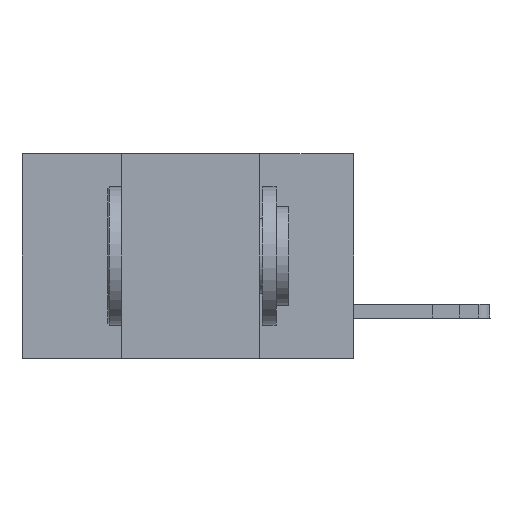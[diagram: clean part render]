
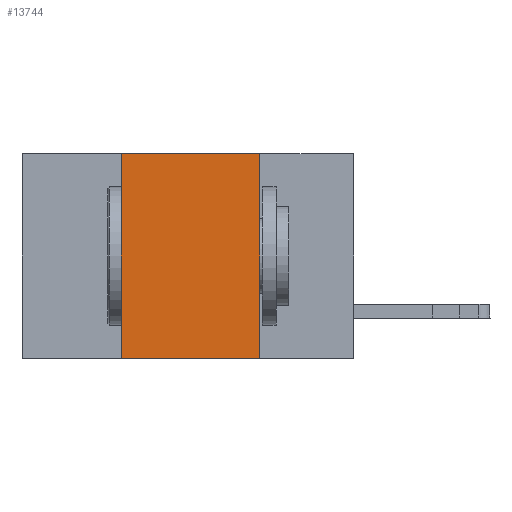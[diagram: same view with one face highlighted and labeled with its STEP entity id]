
A CAD part, left-side view. The second image highlights one B-rep face of the part: STEP entity #13744.
In plain terms, the highlighted planar face has unit normal (-1, 0, 0).
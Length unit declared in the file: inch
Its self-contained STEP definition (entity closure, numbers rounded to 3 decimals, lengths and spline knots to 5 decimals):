
#202 = VECTOR ( 'NONE', #1942, 39.37008 ) ;
#573 = VERTEX_POINT ( 'NONE', #10098 ) ;
#1404 = VECTOR ( 'NONE', #19814, 39.37008 ) ;
#1531 = DIRECTION ( 'NONE',  ( 0., 0., -1. ) ) ;
#1942 = DIRECTION ( 'NONE',  ( 0., 0., -1. ) ) ;
#2146 = LINE ( 'NONE', #12635, #4744 ) ;
#2466 = AXIS2_PLACEMENT_3D ( 'NONE', #9143, #10823, #1531 ) ;
#3136 = CARTESIAN_POINT ( 'NONE',  ( 0., 0.42, -0.37 ) ) ;
#3444 = EDGE_CURVE ( 'NONE', #18048, #16269, #6914, .T. ) ;
#4387 = LINE ( 'NONE', #14983, #10400 ) ;
#4631 = ORIENTED_EDGE ( 'NONE', *, *, #19738, .T. ) ;
#4744 = VECTOR ( 'NONE', #8029, 39.37008 ) ;
#5873 = CARTESIAN_POINT ( 'NONE',  ( 0., 0.17, -0.37 ) ) ;
#6330 = EDGE_LOOP ( 'NONE', ( #6530, #17542, #15235, #4631 ) ) ;
#6530 = ORIENTED_EDGE ( 'NONE', *, *, #3444, .F. ) ;
#6914 = LINE ( 'NONE', #7979, #202 ) ;
#7875 = VERTEX_POINT ( 'NONE', #3136 ) ;
#7979 = CARTESIAN_POINT ( 'NONE',  ( 0., 0.17, 0. ) ) ;
#8029 = DIRECTION ( 'NONE',  ( 0., -1., 0. ) ) ;
#8415 = EDGE_CURVE ( 'NONE', #7875, #573, #16082, .T. ) ;
#9143 = CARTESIAN_POINT ( 'NONE',  ( 0., 0.6, 0. ) ) ;
#10098 = CARTESIAN_POINT ( 'NONE',  ( 0., 0.42, 0. ) ) ;
#10400 = VECTOR ( 'NONE', #19043, 39.37008 ) ;
#10776 = CARTESIAN_POINT ( 'NONE',  ( 0., 0.17, 0. ) ) ;
#10823 = DIRECTION ( 'NONE',  ( 1., 0., 0. ) ) ;
#11269 = FACE_OUTER_BOUND ( 'NONE', #6330, .T. ) ;
#12635 = CARTESIAN_POINT ( 'NONE',  ( 0., 0.6, -0.37 ) ) ;
#13744 = ADVANCED_FACE ( 'NONE', ( #11269 ), #16877, .F. ) ;
#14983 = CARTESIAN_POINT ( 'NONE',  ( 0., 0.6, 0. ) ) ;
#15066 = CARTESIAN_POINT ( 'NONE',  ( 0., 0.42, 0. ) ) ;
#15235 = ORIENTED_EDGE ( 'NONE', *, *, #8415, .F. ) ;
#16082 = LINE ( 'NONE', #15066, #1404 ) ;
#16269 = VERTEX_POINT ( 'NONE', #5873 ) ;
#16877 = PLANE ( 'NONE',  #2466 ) ;
#17391 = EDGE_CURVE ( 'NONE', #573, #18048, #4387, .T. ) ;
#17542 = ORIENTED_EDGE ( 'NONE', *, *, #17391, .F. ) ;
#18048 = VERTEX_POINT ( 'NONE', #10776 ) ;
#19043 = DIRECTION ( 'NONE',  ( 0., -1., 0. ) ) ;
#19738 = EDGE_CURVE ( 'NONE', #7875, #16269, #2146, .T. ) ;
#19814 = DIRECTION ( 'NONE',  ( 0., 0., 1. ) ) ;
